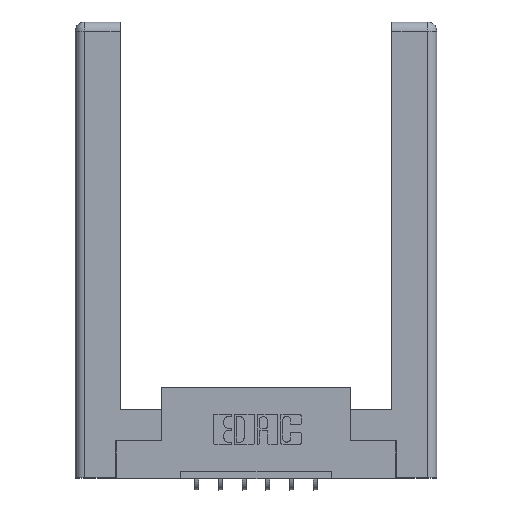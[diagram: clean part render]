
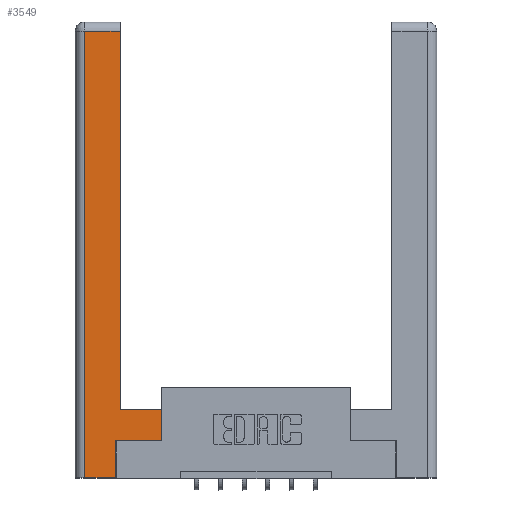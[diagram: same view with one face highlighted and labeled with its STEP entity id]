
A CAD part, top view. The second image highlights one B-rep face of the part: STEP entity #3549.
In plain terms, the highlighted planar face has unit normal (0, 0, 1).
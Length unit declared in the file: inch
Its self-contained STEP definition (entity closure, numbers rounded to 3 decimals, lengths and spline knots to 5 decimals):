
#43 = ORIENTED_EDGE ( 'NONE', *, *, #7861, .T. ) ;
#139 = CARTESIAN_POINT ( 'NONE',  ( 0.265, 0.245, 0. ) ) ;
#172 = EDGE_CURVE ( 'NONE', #10098, #7846, #5142, .T. ) ;
#248 = VECTOR ( 'NONE', #7983, 39.37008 ) ;
#646 = CARTESIAN_POINT ( 'NONE',  ( 0.565, 0.45, 0. ) ) ;
#827 = ORIENTED_EDGE ( 'NONE', *, *, #8416, .T. ) ;
#1061 = VECTOR ( 'NONE', #5373, 39.37008 ) ;
#1065 = AXIS2_PLACEMENT_3D ( 'NONE', #9973, #4568, #6253 ) ;
#1119 = CARTESIAN_POINT ( 'NONE',  ( 0.265, 0., 0. ) ) ;
#1559 = ORIENTED_EDGE ( 'NONE', *, *, #3704, .T. ) ;
#1693 = PLANE ( 'NONE',  #1065 ) ;
#1963 = DIRECTION ( 'NONE',  ( 0., 1., 0. ) ) ;
#2023 = DIRECTION ( 'NONE',  ( 0., 1., 0. ) ) ;
#2508 = VECTOR ( 'NONE', #1963, 39.37008 ) ;
#2530 = FACE_OUTER_BOUND ( 'NONE', #10309, .T. ) ;
#2662 = CARTESIAN_POINT ( 'NONE',  ( 0.565, 0.245, 0. ) ) ;
#3191 = VECTOR ( 'NONE', #6007, 39.37008 ) ;
#3235 = CARTESIAN_POINT ( 'NONE',  ( 0.0615, 2.94, 0. ) ) ;
#3483 = LINE ( 'NONE', #3235, #3191 ) ;
#3549 = ADVANCED_FACE ( 'NONE', ( #2530 ), #1693, .F. ) ;
#3704 = EDGE_CURVE ( 'NONE', #7846, #4244, #10802, .T. ) ;
#3806 = DIRECTION ( 'NONE',  ( 1., 0., 0. ) ) ;
#3950 = LINE ( 'NONE', #11041, #2508 ) ;
#4244 = VERTEX_POINT ( 'NONE', #5956 ) ;
#4533 = ORIENTED_EDGE ( 'NONE', *, *, #11688, .T. ) ;
#4568 = DIRECTION ( 'NONE',  ( 0., 0., -1. ) ) ;
#4757 = CARTESIAN_POINT ( 'NONE',  ( 0.565, 0.45, 0. ) ) ;
#5142 = LINE ( 'NONE', #1119, #9551 ) ;
#5373 = DIRECTION ( 'NONE',  ( 0., -1., 0. ) ) ;
#5566 = LINE ( 'NONE', #9017, #1061 ) ;
#5597 = LINE ( 'NONE', #4757, #8605 ) ;
#5694 = DIRECTION ( 'NONE',  ( 0., 1., 0. ) ) ;
#5701 = VECTOR ( 'NONE', #9492, 39.37008 ) ;
#5768 = CARTESIAN_POINT ( 'NONE',  ( 0.0615, 0., 0. ) ) ;
#5956 = CARTESIAN_POINT ( 'NONE',  ( 0.265, 0.245, 0. ) ) ;
#6007 = DIRECTION ( 'NONE',  ( -1., 0., 0. ) ) ;
#6081 = CARTESIAN_POINT ( 'NONE',  ( 0.295, 2.94, 0. ) ) ;
#6124 = CARTESIAN_POINT ( 'NONE',  ( 0.0615, 2.94, 0. ) ) ;
#6236 = CARTESIAN_POINT ( 'NONE',  ( 0.565, 0.245, 0. ) ) ;
#6253 = DIRECTION ( 'NONE',  ( -1., 0., 0. ) ) ;
#6719 = LINE ( 'NONE', #6236, #248 ) ;
#6802 = EDGE_CURVE ( 'NONE', #9907, #11406, #3483, .T. ) ;
#7194 = EDGE_CURVE ( 'NONE', #4244, #9276, #6719, .T. ) ;
#7218 = CARTESIAN_POINT ( 'NONE',  ( 0.265, 0., 0. ) ) ;
#7828 = EDGE_CURVE ( 'NONE', #11406, #10098, #5566, .T. ) ;
#7846 = VERTEX_POINT ( 'NONE', #7218 ) ;
#7861 = EDGE_CURVE ( 'NONE', #11154, #9534, #10675, .T. ) ;
#7983 = DIRECTION ( 'NONE',  ( 1., 0., 0. ) ) ;
#8416 = EDGE_CURVE ( 'NONE', #9534, #9907, #3950, .T. ) ;
#8605 = VECTOR ( 'NONE', #5694, 39.37008 ) ;
#8956 = ORIENTED_EDGE ( 'NONE', *, *, #7828, .T. ) ;
#9017 = CARTESIAN_POINT ( 'NONE',  ( 0.0615, 0., 0. ) ) ;
#9276 = VERTEX_POINT ( 'NONE', #2662 ) ;
#9296 = ORIENTED_EDGE ( 'NONE', *, *, #172, .T. ) ;
#9492 = DIRECTION ( 'NONE',  ( -1., 0., 0. ) ) ;
#9534 = VERTEX_POINT ( 'NONE', #10423 ) ;
#9551 = VECTOR ( 'NONE', #3806, 39.37008 ) ;
#9907 = VERTEX_POINT ( 'NONE', #6081 ) ;
#9973 = CARTESIAN_POINT ( 'NONE',  ( 0., 0., 0. ) ) ;
#10098 = VERTEX_POINT ( 'NONE', #5768 ) ;
#10309 = EDGE_LOOP ( 'NONE', ( #827, #10455, #8956, #9296, #1559, #10516, #4533, #43 ) ) ;
#10423 = CARTESIAN_POINT ( 'NONE',  ( 0.295, 0.45, 0. ) ) ;
#10455 = ORIENTED_EDGE ( 'NONE', *, *, #6802, .T. ) ;
#10516 = ORIENTED_EDGE ( 'NONE', *, *, #7194, .T. ) ;
#10528 = VECTOR ( 'NONE', #2023, 39.37008 ) ;
#10675 = LINE ( 'NONE', #10840, #5701 ) ;
#10802 = LINE ( 'NONE', #139, #10528 ) ;
#10840 = CARTESIAN_POINT ( 'NONE',  ( 0.295, 0.45, 0. ) ) ;
#11041 = CARTESIAN_POINT ( 'NONE',  ( 0.295, 3., 0. ) ) ;
#11154 = VERTEX_POINT ( 'NONE', #646 ) ;
#11406 = VERTEX_POINT ( 'NONE', #6124 ) ;
#11688 = EDGE_CURVE ( 'NONE', #9276, #11154, #5597, .T. ) ;
